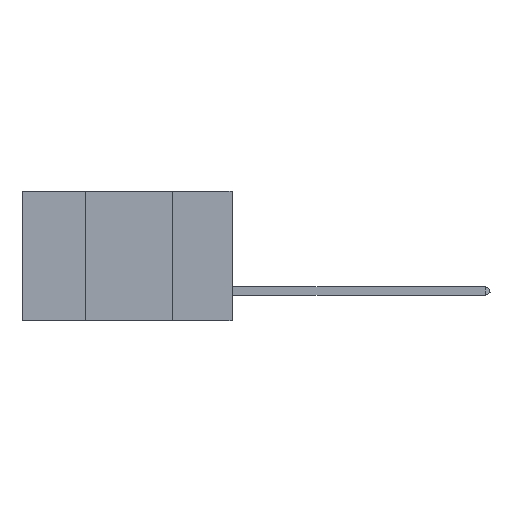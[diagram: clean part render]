
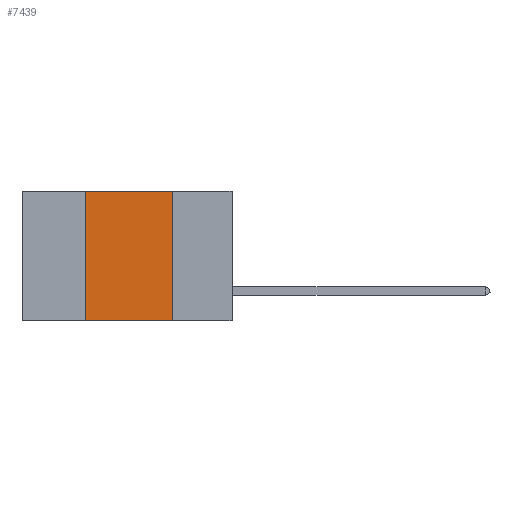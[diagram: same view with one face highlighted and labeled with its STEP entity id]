
A CAD part, left-side view. The second image highlights one B-rep face of the part: STEP entity #7439.
In plain terms, the highlighted planar face has unit normal (-1, 0, 0).
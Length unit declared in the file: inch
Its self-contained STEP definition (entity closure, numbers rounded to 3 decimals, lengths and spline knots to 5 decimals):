
#266 = DIRECTION ( 'NONE',  ( 0., 0., -1. ) ) ;
#1249 = CARTESIAN_POINT ( 'NONE',  ( 0., 0.42, 0. ) ) ;
#1376 = LINE ( 'NONE', #20401, #5644 ) ;
#2718 = FACE_OUTER_BOUND ( 'NONE', #18083, .T. ) ;
#4117 = PLANE ( 'NONE',  #8630 ) ;
#5576 = EDGE_CURVE ( 'NONE', #21087, #6139, #22646, .T. ) ;
#5644 = VECTOR ( 'NONE', #10840, 39.37008 ) ;
#5754 = DIRECTION ( 'NONE',  ( 0., -1., 0. ) ) ;
#5778 = DIRECTION ( 'NONE',  ( 0., -1., 0. ) ) ;
#5847 = CARTESIAN_POINT ( 'NONE',  ( 0., 0.17, -0.37 ) ) ;
#6139 = VERTEX_POINT ( 'NONE', #21317 ) ;
#6365 = VERTEX_POINT ( 'NONE', #13219 ) ;
#7137 = LINE ( 'NONE', #13379, #18538 ) ;
#7439 = ADVANCED_FACE ( 'NONE', ( #2718 ), #4117, .F. ) ;
#7996 = ORIENTED_EDGE ( 'NONE', *, *, #15116, .T. ) ;
#8630 = AXIS2_PLACEMENT_3D ( 'NONE', #21305, #19465, #266 ) ;
#8762 = DIRECTION ( 'NONE',  ( 0., 0., 1. ) ) ;
#9415 = ORIENTED_EDGE ( 'NONE', *, *, #15320, .F. ) ;
#10840 = DIRECTION ( 'NONE',  ( 0., 0., -1. ) ) ;
#11554 = CARTESIAN_POINT ( 'NONE',  ( 0., 0.42, -0.37 ) ) ;
#12349 = VECTOR ( 'NONE', #5754, 39.37008 ) ;
#12754 = EDGE_CURVE ( 'NONE', #6139, #6365, #20764, .T. ) ;
#13219 = CARTESIAN_POINT ( 'NONE',  ( 0., 0.17, 0. ) ) ;
#13379 = CARTESIAN_POINT ( 'NONE',  ( 0., 0.6, -0.37 ) ) ;
#15116 = EDGE_CURVE ( 'NONE', #21087, #19105, #7137, .T. ) ;
#15320 = EDGE_CURVE ( 'NONE', #6365, #19105, #1376, .T. ) ;
#18083 = EDGE_LOOP ( 'NONE', ( #9415, #20493, #23024, #7996 ) ) ;
#18538 = VECTOR ( 'NONE', #5778, 39.37008 ) ;
#19105 = VERTEX_POINT ( 'NONE', #5847 ) ;
#19465 = DIRECTION ( 'NONE',  ( 1., 0., 0. ) ) ;
#20401 = CARTESIAN_POINT ( 'NONE',  ( 0., 0.17, 0. ) ) ;
#20493 = ORIENTED_EDGE ( 'NONE', *, *, #12754, .F. ) ;
#20764 = LINE ( 'NONE', #24630, #12349 ) ;
#21087 = VERTEX_POINT ( 'NONE', #11554 ) ;
#21305 = CARTESIAN_POINT ( 'NONE',  ( 0., 0.6, 0. ) ) ;
#21317 = CARTESIAN_POINT ( 'NONE',  ( 0., 0.42, 0. ) ) ;
#22646 = LINE ( 'NONE', #1249, #24150 ) ;
#23024 = ORIENTED_EDGE ( 'NONE', *, *, #5576, .F. ) ;
#24150 = VECTOR ( 'NONE', #8762, 39.37008 ) ;
#24630 = CARTESIAN_POINT ( 'NONE',  ( 0., 0.6, 0. ) ) ;
